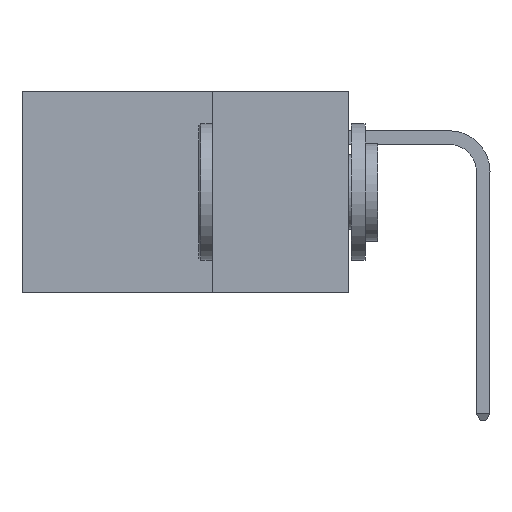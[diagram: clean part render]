
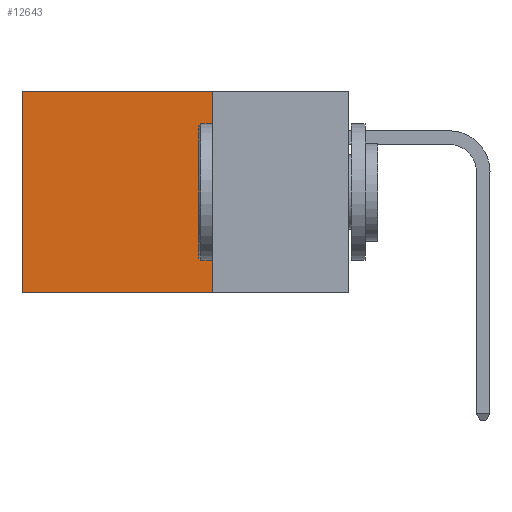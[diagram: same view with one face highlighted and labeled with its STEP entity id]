
A CAD part, left-side view. The second image highlights one B-rep face of the part: STEP entity #12643.
In plain terms, the highlighted planar face has unit normal (-1, 0, 0).
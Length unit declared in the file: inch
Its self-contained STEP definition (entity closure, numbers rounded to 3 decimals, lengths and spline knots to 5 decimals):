
#383 = DIRECTION ( 'NONE',  ( 0., 0., -1. ) ) ;
#2010 = DIRECTION ( 'NONE',  ( 0., 1., 0. ) ) ;
#3037 = VERTEX_POINT ( 'NONE', #21583 ) ;
#3750 = CARTESIAN_POINT ( 'NONE',  ( 0.2875, 0.25, 0. ) ) ;
#4125 = DIRECTION ( 'NONE',  ( 0., 0., -1. ) ) ;
#4339 = LINE ( 'NONE', #25356, #15558 ) ;
#4939 = LINE ( 'NONE', #16196, #10916 ) ;
#7116 = DIRECTION ( 'NONE',  ( 0., 1., 0. ) ) ;
#7225 = PLANE ( 'NONE',  #18936 ) ;
#7917 = DIRECTION ( 'NONE',  ( 0., 0., -1. ) ) ;
#9642 = CARTESIAN_POINT ( 'NONE',  ( 0.2875, 0.25, -0.37 ) ) ;
#9765 = EDGE_CURVE ( 'NONE', #14947, #18711, #24856, .T. ) ;
#10655 = ORIENTED_EDGE ( 'NONE', *, *, #26472, .F. ) ;
#10916 = VECTOR ( 'NONE', #7116, 39.37008 ) ;
#12643 = ADVANCED_FACE ( 'NONE', ( #22952 ), #7225, .F. ) ;
#12967 = CARTESIAN_POINT ( 'NONE',  ( 0.2875, 0.6, -0.37 ) ) ;
#13248 = ORIENTED_EDGE ( 'NONE', *, *, #16749, .T. ) ;
#13936 = DIRECTION ( 'NONE',  ( 1., 0., 0. ) ) ;
#14320 = VECTOR ( 'NONE', #4125, 39.37008 ) ;
#14595 = EDGE_CURVE ( 'NONE', #14947, #3037, #4939, .T. ) ;
#14947 = VERTEX_POINT ( 'NONE', #3750 ) ;
#15558 = VECTOR ( 'NONE', #2010, 39.37008 ) ;
#16196 = CARTESIAN_POINT ( 'NONE',  ( 0.2875, 0.25, 0. ) ) ;
#16749 = EDGE_CURVE ( 'NONE', #3037, #16919, #23074, .T. ) ;
#16919 = VERTEX_POINT ( 'NONE', #12967 ) ;
#17586 = CARTESIAN_POINT ( 'NONE',  ( 0.2875, 0.25, 0. ) ) ;
#18711 = VERTEX_POINT ( 'NONE', #9642 ) ;
#18936 = AXIS2_PLACEMENT_3D ( 'NONE', #27428, #13936, #383 ) ;
#21319 = CARTESIAN_POINT ( 'NONE',  ( 0.2875, 0.6, 0. ) ) ;
#21583 = CARTESIAN_POINT ( 'NONE',  ( 0.2875, 0.6, 0. ) ) ;
#22952 = FACE_OUTER_BOUND ( 'NONE', #27328, .T. ) ;
#22970 = ORIENTED_EDGE ( 'NONE', *, *, #9765, .F. ) ;
#23074 = LINE ( 'NONE', #21319, #28379 ) ;
#23268 = ORIENTED_EDGE ( 'NONE', *, *, #14595, .T. ) ;
#24856 = LINE ( 'NONE', #17586, #14320 ) ;
#25356 = CARTESIAN_POINT ( 'NONE',  ( 0.2875, 0.25, -0.37 ) ) ;
#26472 = EDGE_CURVE ( 'NONE', #18711, #16919, #4339, .T. ) ;
#27328 = EDGE_LOOP ( 'NONE', ( #13248, #10655, #22970, #23268 ) ) ;
#27428 = CARTESIAN_POINT ( 'NONE',  ( 0.2875, 0.25, 0. ) ) ;
#28379 = VECTOR ( 'NONE', #7917, 39.37008 ) ;
